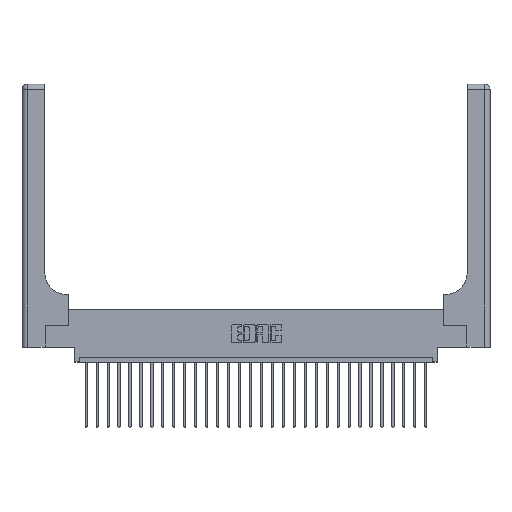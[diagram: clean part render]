
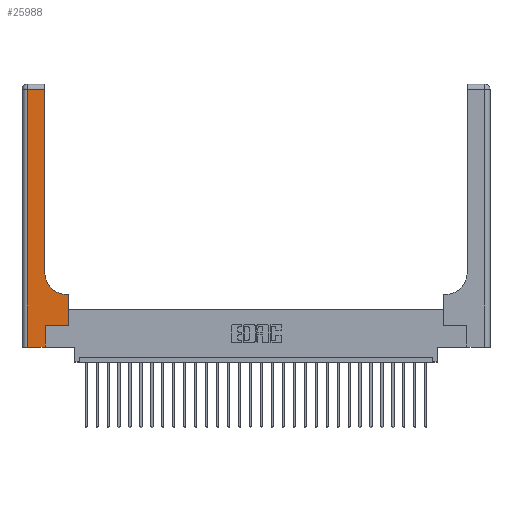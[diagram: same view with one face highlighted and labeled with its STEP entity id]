
A CAD part, top view. The second image highlights one B-rep face of the part: STEP entity #25988.
In plain terms, the highlighted planar face has unit normal (0, 0, 1).
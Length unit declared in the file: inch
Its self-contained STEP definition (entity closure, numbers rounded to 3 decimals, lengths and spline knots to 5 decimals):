
#227 = CARTESIAN_POINT ( 'NONE',  ( 0.528, 0.25, 0.37 ) ) ;
#355 = VECTOR ( 'NONE', #5038, 39.37008 ) ;
#411 = PLANE ( 'NONE',  #6887 ) ;
#1042 = LINE ( 'NONE', #7454, #20590 ) ;
#1423 = VECTOR ( 'NONE', #25265, 39.37008 ) ;
#1426 = DIRECTION ( 'NONE',  ( 0., 1., 0. ) ) ;
#1605 = EDGE_CURVE ( 'NONE', #7632, #16102, #22053, .T. ) ;
#2128 = CARTESIAN_POINT ( 'NONE',  ( 0., 3., 0.37 ) ) ;
#2313 = DIRECTION ( 'NONE',  ( 0., 1., 0. ) ) ;
#3042 = VECTOR ( 'NONE', #14514, 39.37008 ) ;
#3113 = CARTESIAN_POINT ( 'NONE',  ( 0.528, 0.6, 0.37 ) ) ;
#3356 = LINE ( 'NONE', #12457, #3042 ) ;
#3958 = AXIS2_PLACEMENT_3D ( 'NONE', #13626, #15694, #8513 ) ;
#4064 = DIRECTION ( 'NONE',  ( -1., 0., 0. ) ) ;
#4684 = LINE ( 'NONE', #10980, #1423 ) ;
#5038 = DIRECTION ( 'NONE',  ( 0., -1., 0. ) ) ;
#5288 = VERTEX_POINT ( 'NONE', #19718 ) ;
#6740 = ORIENTED_EDGE ( 'NONE', *, *, #9522, .T. ) ;
#6769 = ORIENTED_EDGE ( 'NONE', *, *, #21614, .T. ) ;
#6887 = AXIS2_PLACEMENT_3D ( 'NONE', #2128, #10387, #16483 ) ;
#6947 = ORIENTED_EDGE ( 'NONE', *, *, #9639, .T. ) ;
#7059 = ORIENTED_EDGE ( 'NONE', *, *, #26029, .T. ) ;
#7236 = EDGE_CURVE ( 'NONE', #22329, #11062, #14653, .T. ) ;
#7454 = CARTESIAN_POINT ( 'NONE',  ( 0.265, 0., 0.37 ) ) ;
#7632 = VERTEX_POINT ( 'NONE', #25588 ) ;
#8513 = DIRECTION ( 'NONE',  ( 1., 0., 0. ) ) ;
#8685 = CARTESIAN_POINT ( 'NONE',  ( 0.51, 0.6, 0.37 ) ) ;
#8864 = EDGE_CURVE ( 'NONE', #5288, #7632, #15062, .T. ) ;
#9024 = CARTESIAN_POINT ( 'NONE',  ( 0.265, 0.25, 0.37 ) ) ;
#9522 = EDGE_CURVE ( 'NONE', #14642, #22329, #9628, .T. ) ;
#9628 = LINE ( 'NONE', #227, #12861 ) ;
#9639 = EDGE_CURVE ( 'NONE', #11062, #5288, #26258, .T. ) ;
#9879 = VECTOR ( 'NONE', #4064, 39.37008 ) ;
#9949 = DIRECTION ( 'NONE',  ( -1., 0., 0. ) ) ;
#10387 = DIRECTION ( 'NONE',  ( 0., 0., -1. ) ) ;
#10473 = VECTOR ( 'NONE', #9949, 39.37008 ) ;
#10774 = ORIENTED_EDGE ( 'NONE', *, *, #13212, .T. ) ;
#10980 = CARTESIAN_POINT ( 'NONE',  ( 0.265, 0.25, 0.37 ) ) ;
#11039 = CARTESIAN_POINT ( 'NONE',  ( 0.528, 0.25, 0.37 ) ) ;
#11062 = VERTEX_POINT ( 'NONE', #8685 ) ;
#11600 = CARTESIAN_POINT ( 'NONE',  ( 0.265, 0., 0.37 ) ) ;
#11971 = EDGE_LOOP ( 'NONE', ( #22438, #23313, #6769, #7059, #16864, #10774, #6740, #12766, #6947 ) ) ;
#12255 = LINE ( 'NONE', #12907, #355 ) ;
#12457 = CARTESIAN_POINT ( 'NONE',  ( 0., 0., 0.37 ) ) ;
#12712 = VERTEX_POINT ( 'NONE', #17380 ) ;
#12766 = ORIENTED_EDGE ( 'NONE', *, *, #7236, .T. ) ;
#12861 = VECTOR ( 'NONE', #2313, 39.37008 ) ;
#12907 = CARTESIAN_POINT ( 'NONE',  ( 0.06, 3., 0.37 ) ) ;
#13212 = EDGE_CURVE ( 'NONE', #13599, #14642, #4684, .T. ) ;
#13599 = VERTEX_POINT ( 'NONE', #9024 ) ;
#13626 = CARTESIAN_POINT ( 'NONE',  ( 0.51, 0.85, 0.37 ) ) ;
#14514 = DIRECTION ( 'NONE',  ( 1., 0., 0. ) ) ;
#14642 = VERTEX_POINT ( 'NONE', #11039 ) ;
#14653 = LINE ( 'NONE', #19470, #10473 ) ;
#14981 = VECTOR ( 'NONE', #22037, 39.37008 ) ;
#15062 = LINE ( 'NONE', #19572, #14981 ) ;
#15694 = DIRECTION ( 'NONE',  ( 0., 0., -1. ) ) ;
#16102 = VERTEX_POINT ( 'NONE', #16254 ) ;
#16254 = CARTESIAN_POINT ( 'NONE',  ( 0.06, 2.94, 0.37 ) ) ;
#16483 = DIRECTION ( 'NONE',  ( -1., 0., 0. ) ) ;
#16864 = ORIENTED_EDGE ( 'NONE', *, *, #21190, .T. ) ;
#17380 = CARTESIAN_POINT ( 'NONE',  ( 0.06, 0., 0.37 ) ) ;
#19061 = FACE_OUTER_BOUND ( 'NONE', #11971, .T. ) ;
#19085 = VERTEX_POINT ( 'NONE', #11600 ) ;
#19470 = CARTESIAN_POINT ( 'NONE',  ( 0.26, 0.6, 0.37 ) ) ;
#19572 = CARTESIAN_POINT ( 'NONE',  ( 0.26, 3., 0.37 ) ) ;
#19718 = CARTESIAN_POINT ( 'NONE',  ( 0.26, 0.85, 0.37 ) ) ;
#20590 = VECTOR ( 'NONE', #1426, 39.37008 ) ;
#21190 = EDGE_CURVE ( 'NONE', #19085, #13599, #1042, .T. ) ;
#21614 = EDGE_CURVE ( 'NONE', #16102, #12712, #12255, .T. ) ;
#22037 = DIRECTION ( 'NONE',  ( 0., 1., 0. ) ) ;
#22053 = LINE ( 'NONE', #26317, #9879 ) ;
#22329 = VERTEX_POINT ( 'NONE', #3113 ) ;
#22438 = ORIENTED_EDGE ( 'NONE', *, *, #8864, .T. ) ;
#23313 = ORIENTED_EDGE ( 'NONE', *, *, #1605, .T. ) ;
#25265 = DIRECTION ( 'NONE',  ( 1., 0., 0. ) ) ;
#25588 = CARTESIAN_POINT ( 'NONE',  ( 0.26, 2.94, 0.37 ) ) ;
#25988 = ADVANCED_FACE ( 'NONE', ( #19061 ), #411, .F. ) ;
#26029 = EDGE_CURVE ( 'NONE', #12712, #19085, #3356, .T. ) ;
#26258 = CIRCLE ( 'NONE', #3958, 0.25 ) ;
#26317 = CARTESIAN_POINT ( 'NONE',  ( 0., 2.94, 0.37 ) ) ;
